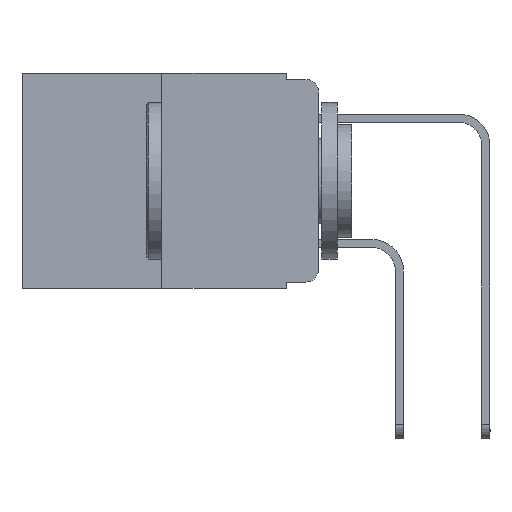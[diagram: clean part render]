
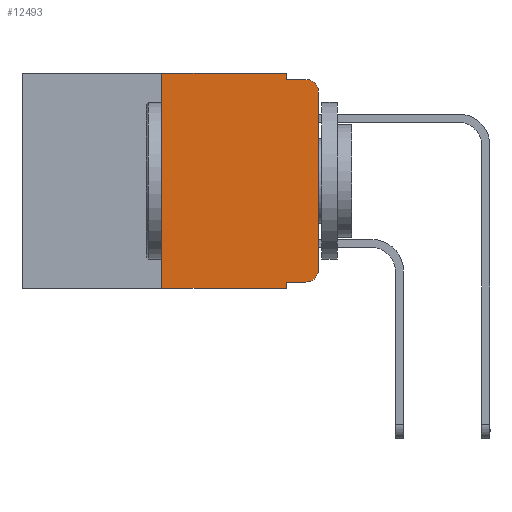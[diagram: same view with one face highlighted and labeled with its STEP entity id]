
A CAD part, left-side view. The second image highlights one B-rep face of the part: STEP entity #12493.
In plain terms, the highlighted planar face has unit normal (-1, 0, 0).
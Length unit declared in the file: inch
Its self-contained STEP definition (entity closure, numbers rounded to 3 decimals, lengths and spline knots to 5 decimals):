
#263 = VECTOR ( 'NONE', #9170, 39.37008 ) ;
#640 = DIRECTION ( 'NONE',  ( 0., 0., 1. ) ) ;
#774 = FACE_OUTER_BOUND ( 'NONE', #4221, .T. ) ;
#889 = LINE ( 'NONE', #4018, #11535 ) ;
#892 = CARTESIAN_POINT ( 'NONE',  ( 0., 0.051, 0. ) ) ;
#905 = EDGE_CURVE ( 'NONE', #5258, #4361, #11947, .T. ) ;
#953 = CARTESIAN_POINT ( 'NONE',  ( 0., 0.051, -0.01 ) ) ;
#1022 = CARTESIAN_POINT ( 'NONE',  ( 0., 0.25, -0.343 ) ) ;
#1540 = VECTOR ( 'NONE', #14755, 39.37008 ) ;
#1663 = ORIENTED_EDGE ( 'NONE', *, *, #2150, .T. ) ;
#1715 = EDGE_CURVE ( 'NONE', #13713, #2564, #6386, .T. ) ;
#2150 = EDGE_CURVE ( 'NONE', #16400, #5258, #6590, .T. ) ;
#2284 = AXIS2_PLACEMENT_3D ( 'NONE', #2499, #15620, #14368 ) ;
#2396 = VERTEX_POINT ( 'NONE', #7993 ) ;
#2499 = CARTESIAN_POINT ( 'NONE',  ( 0., 0.473, 0. ) ) ;
#2564 = VERTEX_POINT ( 'NONE', #11408 ) ;
#2651 = DIRECTION ( 'NONE',  ( 0., -1., 0. ) ) ;
#2661 = DIRECTION ( 'NONE',  ( -1., 0., 0. ) ) ;
#2810 = ORIENTED_EDGE ( 'NONE', *, *, #7475, .F. ) ;
#2848 = ORIENTED_EDGE ( 'NONE', *, *, #7305, .T. ) ;
#2854 = EDGE_CURVE ( 'NONE', #2396, #16400, #8400, .T. ) ;
#3861 = ORIENTED_EDGE ( 'NONE', *, *, #12092, .T. ) ;
#3871 = CARTESIAN_POINT ( 'NONE',  ( 0., 0.051, -0.333 ) ) ;
#3908 = VECTOR ( 'NONE', #640, 39.37008 ) ;
#4003 = ORIENTED_EDGE ( 'NONE', *, *, #9547, .F. ) ;
#4018 = CARTESIAN_POINT ( 'NONE',  ( 0., 0.473, 0. ) ) ;
#4028 = DIRECTION ( 'NONE',  ( 0., -1., 0. ) ) ;
#4221 = EDGE_LOOP ( 'NONE', ( #1663, #6124, #15171, #15452, #4003, #7267, #3861, #2810, #2848, #14379 ) ) ;
#4361 = VERTEX_POINT ( 'NONE', #11724 ) ;
#4690 = EDGE_CURVE ( 'NONE', #10012, #4361, #11651, .T. ) ;
#4708 = CARTESIAN_POINT ( 'NONE',  ( 0., 0.25, 0. ) ) ;
#4873 = DIRECTION ( 'NONE',  ( -1., 0., 0. ) ) ;
#5191 = DIRECTION ( 'NONE',  ( 0., -1., 0. ) ) ;
#5258 = VERTEX_POINT ( 'NONE', #11818 ) ;
#5653 = LINE ( 'NONE', #9234, #16329 ) ;
#5976 = VERTEX_POINT ( 'NONE', #3871 ) ;
#6101 = CARTESIAN_POINT ( 'NONE',  ( 0., 0.051, -0.01 ) ) ;
#6124 = ORIENTED_EDGE ( 'NONE', *, *, #905, .T. ) ;
#6386 = LINE ( 'NONE', #4708, #3908 ) ;
#6590 = LINE ( 'NONE', #10481, #263 ) ;
#6632 = CARTESIAN_POINT ( 'NONE',  ( 0., 0.02, -0.313 ) ) ;
#7010 = AXIS2_PLACEMENT_3D ( 'NONE', #6632, #2661, #13176 ) ;
#7267 = ORIENTED_EDGE ( 'NONE', *, *, #1715, .F. ) ;
#7305 = EDGE_CURVE ( 'NONE', #5976, #2396, #16486, .T. ) ;
#7475 = EDGE_CURVE ( 'NONE', #5976, #15778, #15667, .T. ) ;
#7604 = PLANE ( 'NONE',  #2284 ) ;
#7993 = CARTESIAN_POINT ( 'NONE',  ( 0., 0.02, -0.333 ) ) ;
#8140 = VECTOR ( 'NONE', #8942, 39.37008 ) ;
#8400 = CIRCLE ( 'NONE', #7010, 0.02 ) ;
#8942 = DIRECTION ( 'NONE',  ( 0., -1., 0. ) ) ;
#9102 = CARTESIAN_POINT ( 'NONE',  ( 0., 0.051, -0.333 ) ) ;
#9149 = VECTOR ( 'NONE', #14163, 39.37008 ) ;
#9170 = DIRECTION ( 'NONE',  ( 0., 0., 1. ) ) ;
#9234 = CARTESIAN_POINT ( 'NONE',  ( 0., 0.473, -0.343 ) ) ;
#9547 = EDGE_CURVE ( 'NONE', #2564, #11915, #889, .T. ) ;
#9649 = CARTESIAN_POINT ( 'NONE',  ( 0., 0., -0.313 ) ) ;
#10012 = VERTEX_POINT ( 'NONE', #6101 ) ;
#10138 = DIRECTION ( 'NONE',  ( 0., 0., -1. ) ) ;
#10380 = CARTESIAN_POINT ( 'NONE',  ( 0., 0.051, 0. ) ) ;
#10481 = CARTESIAN_POINT ( 'NONE',  ( 0., 0., 0. ) ) ;
#11408 = CARTESIAN_POINT ( 'NONE',  ( 0., 0.25, 0. ) ) ;
#11535 = VECTOR ( 'NONE', #2651, 39.37008 ) ;
#11651 = LINE ( 'NONE', #953, #8140 ) ;
#11724 = CARTESIAN_POINT ( 'NONE',  ( 0., 0.02, -0.01 ) ) ;
#11818 = CARTESIAN_POINT ( 'NONE',  ( 0., 0., -0.03 ) ) ;
#11915 = VERTEX_POINT ( 'NONE', #892 ) ;
#11947 = CIRCLE ( 'NONE', #16800, 0.02 ) ;
#12092 = EDGE_CURVE ( 'NONE', #13713, #15778, #5653, .T. ) ;
#12493 = ADVANCED_FACE ( 'NONE', ( #774 ), #7604, .F. ) ;
#12619 = VECTOR ( 'NONE', #4028, 39.37008 ) ;
#13176 = DIRECTION ( 'NONE',  ( 0., 0., -1. ) ) ;
#13239 = CARTESIAN_POINT ( 'NONE',  ( 0., 0.051, -0.343 ) ) ;
#13713 = VERTEX_POINT ( 'NONE', #1022 ) ;
#13839 = EDGE_CURVE ( 'NONE', #11915, #10012, #16499, .T. ) ;
#14163 = DIRECTION ( 'NONE',  ( 0., 0., -1. ) ) ;
#14368 = DIRECTION ( 'NONE',  ( 0., 0., -1. ) ) ;
#14379 = ORIENTED_EDGE ( 'NONE', *, *, #2854, .T. ) ;
#14755 = DIRECTION ( 'NONE',  ( 0., 0., -1. ) ) ;
#14805 = CARTESIAN_POINT ( 'NONE',  ( 0., 0.051, 0. ) ) ;
#15171 = ORIENTED_EDGE ( 'NONE', *, *, #4690, .F. ) ;
#15449 = CARTESIAN_POINT ( 'NONE',  ( 0., 0.02, -0.03 ) ) ;
#15452 = ORIENTED_EDGE ( 'NONE', *, *, #13839, .F. ) ;
#15620 = DIRECTION ( 'NONE',  ( 1., 0., 0. ) ) ;
#15667 = LINE ( 'NONE', #14805, #1540 ) ;
#15778 = VERTEX_POINT ( 'NONE', #13239 ) ;
#16329 = VECTOR ( 'NONE', #5191, 39.37008 ) ;
#16400 = VERTEX_POINT ( 'NONE', #9649 ) ;
#16486 = LINE ( 'NONE', #9102, #12619 ) ;
#16499 = LINE ( 'NONE', #10380, #9149 ) ;
#16800 = AXIS2_PLACEMENT_3D ( 'NONE', #15449, #4873, #10138 ) ;
